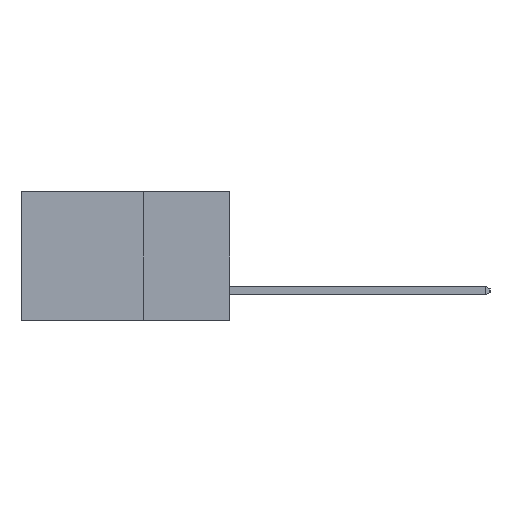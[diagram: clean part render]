
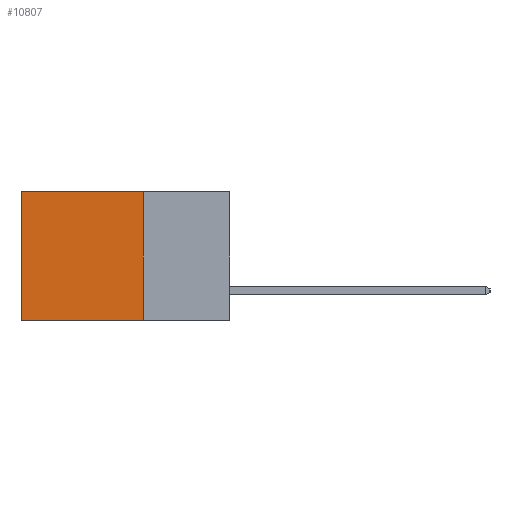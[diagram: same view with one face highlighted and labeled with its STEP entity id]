
A CAD part, left-side view. The second image highlights one B-rep face of the part: STEP entity #10807.
In plain terms, the highlighted planar face has unit normal (-1, 0, 0).
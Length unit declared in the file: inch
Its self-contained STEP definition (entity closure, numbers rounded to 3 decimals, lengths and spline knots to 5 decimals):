
#160 = CARTESIAN_POINT ( 'NONE',  ( 0.2615, 0.6, -0.37 ) ) ;
#598 = DIRECTION ( 'NONE',  ( 0., 1., 0. ) ) ;
#1582 = AXIS2_PLACEMENT_3D ( 'NONE', #4876, #5857, #12911 ) ;
#1876 = LINE ( 'NONE', #10805, #12691 ) ;
#2005 = ORIENTED_EDGE ( 'NONE', *, *, #12231, .T. ) ;
#2144 = LINE ( 'NONE', #12804, #12288 ) ;
#3152 = VERTEX_POINT ( 'NONE', #13098 ) ;
#3394 = EDGE_CURVE ( 'NONE', #5747, #12536, #9145, .T. ) ;
#4533 = FACE_OUTER_BOUND ( 'NONE', #5882, .T. ) ;
#4646 = VECTOR ( 'NONE', #9390, 39.37008 ) ;
#4744 = DIRECTION ( 'NONE',  ( 0., 1., 0. ) ) ;
#4876 = CARTESIAN_POINT ( 'NONE',  ( 0.2615, 0.25, -0.37 ) ) ;
#5450 = CARTESIAN_POINT ( 'NONE',  ( 0.2615, 0.25, 0. ) ) ;
#5747 = VERTEX_POINT ( 'NONE', #5450 ) ;
#5857 = DIRECTION ( 'NONE',  ( 1., 0., 0. ) ) ;
#5882 = EDGE_LOOP ( 'NONE', ( #2005, #6836, #6630, #7126 ) ) ;
#6458 = VECTOR ( 'NONE', #8515, 39.37008 ) ;
#6630 = ORIENTED_EDGE ( 'NONE', *, *, #3394, .F. ) ;
#6836 = ORIENTED_EDGE ( 'NONE', *, *, #9123, .F. ) ;
#6962 = CARTESIAN_POINT ( 'NONE',  ( 0.2615, 0.6, -0.37 ) ) ;
#7126 = ORIENTED_EDGE ( 'NONE', *, *, #11835, .T. ) ;
#7256 = CARTESIAN_POINT ( 'NONE',  ( 0.2615, 0.25, -0.37 ) ) ;
#8515 = DIRECTION ( 'NONE',  ( 0., 0., -1. ) ) ;
#9123 = EDGE_CURVE ( 'NONE', #12536, #12049, #2144, .T. ) ;
#9145 = LINE ( 'NONE', #7256, #6458 ) ;
#9390 = DIRECTION ( 'NONE',  ( 0., 0., -1. ) ) ;
#9855 = CARTESIAN_POINT ( 'NONE',  ( 0.2615, 0.25, -0.37 ) ) ;
#10805 = CARTESIAN_POINT ( 'NONE',  ( 0.2615, 0.25, 0. ) ) ;
#10807 = ADVANCED_FACE ( 'NONE', ( #4533 ), #10915, .F. ) ;
#10915 = PLANE ( 'NONE',  #1582 ) ;
#11835 = EDGE_CURVE ( 'NONE', #5747, #3152, #1876, .T. ) ;
#12049 = VERTEX_POINT ( 'NONE', #6962 ) ;
#12231 = EDGE_CURVE ( 'NONE', #3152, #12049, #12359, .T. ) ;
#12288 = VECTOR ( 'NONE', #598, 39.37008 ) ;
#12359 = LINE ( 'NONE', #160, #4646 ) ;
#12536 = VERTEX_POINT ( 'NONE', #9855 ) ;
#12691 = VECTOR ( 'NONE', #4744, 39.37008 ) ;
#12804 = CARTESIAN_POINT ( 'NONE',  ( 0.2615, 0.25, -0.37 ) ) ;
#12911 = DIRECTION ( 'NONE',  ( 0., 0., -1. ) ) ;
#13098 = CARTESIAN_POINT ( 'NONE',  ( 0.2615, 0.6, 0. ) ) ;
